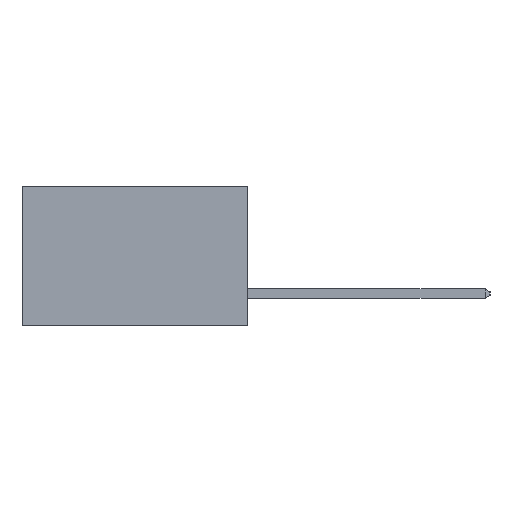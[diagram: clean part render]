
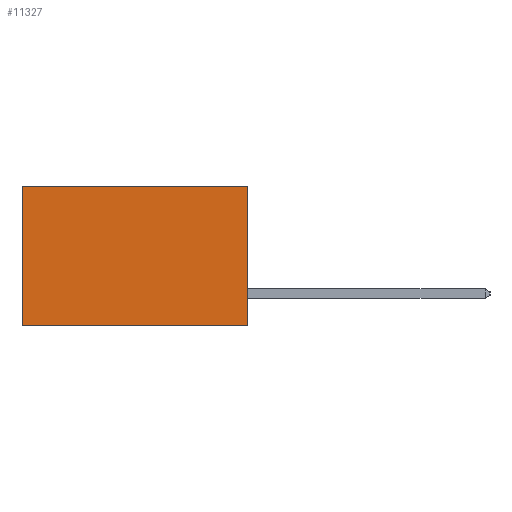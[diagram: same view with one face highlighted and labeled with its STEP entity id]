
A CAD part, left-side view. The second image highlights one B-rep face of the part: STEP entity #11327.
In plain terms, the highlighted planar face has unit normal (-1, 0, 0).
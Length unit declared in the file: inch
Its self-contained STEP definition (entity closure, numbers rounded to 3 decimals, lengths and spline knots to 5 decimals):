
#675 = VECTOR ( 'NONE', #13826, 39.37008 ) ;
#1206 = LINE ( 'NONE', #4774, #675 ) ;
#2151 = EDGE_CURVE ( 'NONE', #11054, #19984, #1206, .T. ) ;
#2547 = CARTESIAN_POINT ( 'NONE',  ( 0.298, 0.6, 0. ) ) ;
#2968 = AXIS2_PLACEMENT_3D ( 'NONE', #6772, #8562, #20649 ) ;
#3616 = ORIENTED_EDGE ( 'NONE', *, *, #8566, .T. ) ;
#4774 = CARTESIAN_POINT ( 'NONE',  ( 0.298, 0., 0. ) ) ;
#5218 = FACE_OUTER_BOUND ( 'NONE', #13389, .T. ) ;
#5235 = LINE ( 'NONE', #8883, #14050 ) ;
#6772 = CARTESIAN_POINT ( 'NONE',  ( 0.298, 0., 0. ) ) ;
#7179 = VECTOR ( 'NONE', #17226, 39.37008 ) ;
#8407 = CARTESIAN_POINT ( 'NONE',  ( 0.298, 0.6, -0.37 ) ) ;
#8562 = DIRECTION ( 'NONE',  ( 1., 0., 0. ) ) ;
#8566 = EDGE_CURVE ( 'NONE', #14254, #20021, #11962, .T. ) ;
#8883 = CARTESIAN_POINT ( 'NONE',  ( 0.298, 0., 0. ) ) ;
#9639 = VECTOR ( 'NONE', #20134, 39.37008 ) ;
#9821 = CARTESIAN_POINT ( 'NONE',  ( 0.298, 0., -0.37 ) ) ;
#10718 = DIRECTION ( 'NONE',  ( 0., 1., 0. ) ) ;
#10894 = EDGE_CURVE ( 'NONE', #11054, #14254, #5235, .T. ) ;
#11054 = VERTEX_POINT ( 'NONE', #16305 ) ;
#11327 = ADVANCED_FACE ( 'NONE', ( #5218 ), #12113, .F. ) ;
#11962 = LINE ( 'NONE', #20387, #7179 ) ;
#12113 = PLANE ( 'NONE',  #2968 ) ;
#13297 = EDGE_CURVE ( 'NONE', #19984, #20021, #14335, .T. ) ;
#13389 = EDGE_LOOP ( 'NONE', ( #3616, #18955, #13393, #17274 ) ) ;
#13393 = ORIENTED_EDGE ( 'NONE', *, *, #2151, .F. ) ;
#13826 = DIRECTION ( 'NONE',  ( 0., 0., -1. ) ) ;
#14050 = VECTOR ( 'NONE', #10718, 39.37008 ) ;
#14254 = VERTEX_POINT ( 'NONE', #2547 ) ;
#14335 = LINE ( 'NONE', #9821, #9639 ) ;
#16305 = CARTESIAN_POINT ( 'NONE',  ( 0.298, 0., 0. ) ) ;
#17226 = DIRECTION ( 'NONE',  ( 0., 0., -1. ) ) ;
#17274 = ORIENTED_EDGE ( 'NONE', *, *, #10894, .T. ) ;
#18725 = CARTESIAN_POINT ( 'NONE',  ( 0.298, 0., -0.37 ) ) ;
#18955 = ORIENTED_EDGE ( 'NONE', *, *, #13297, .F. ) ;
#19984 = VERTEX_POINT ( 'NONE', #18725 ) ;
#20021 = VERTEX_POINT ( 'NONE', #8407 ) ;
#20134 = DIRECTION ( 'NONE',  ( 0., 1., 0. ) ) ;
#20387 = CARTESIAN_POINT ( 'NONE',  ( 0.298, 0.6, 0. ) ) ;
#20649 = DIRECTION ( 'NONE',  ( 0., 0., -1. ) ) ;
